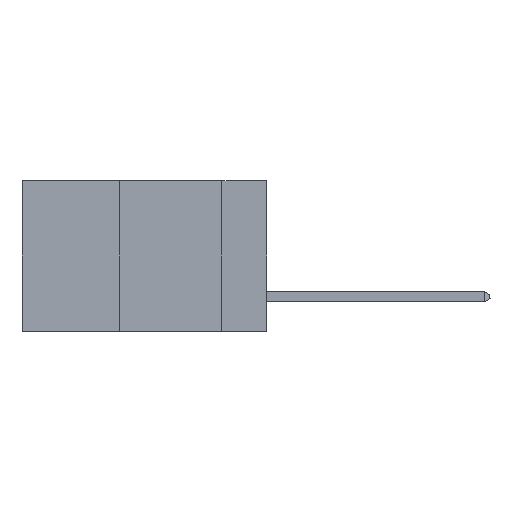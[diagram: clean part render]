
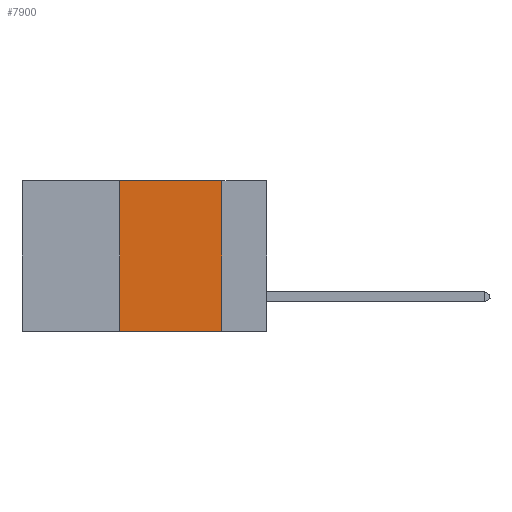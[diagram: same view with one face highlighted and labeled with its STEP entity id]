
A CAD part, left-side view. The second image highlights one B-rep face of the part: STEP entity #7900.
In plain terms, the highlighted planar face has unit normal (-1, 0, 0).
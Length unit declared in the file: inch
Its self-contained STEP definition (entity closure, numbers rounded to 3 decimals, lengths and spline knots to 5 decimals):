
#352 = DIRECTION ( 'NONE',  ( 0., -1., 0. ) ) ;
#360 = ORIENTED_EDGE ( 'NONE', *, *, #14036, .F. ) ;
#533 = LINE ( 'NONE', #4120, #10003 ) ;
#816 = VECTOR ( 'NONE', #3423, 39.37008 ) ;
#871 = EDGE_CURVE ( 'NONE', #8733, #17433, #17259, .T. ) ;
#1996 = CARTESIAN_POINT ( 'NONE',  ( 0., 0.11, 0. ) ) ;
#3182 = LINE ( 'NONE', #10126, #15303 ) ;
#3423 = DIRECTION ( 'NONE',  ( 0., 0., -1. ) ) ;
#3440 = CARTESIAN_POINT ( 'NONE',  ( 0., 0.36, -0.37 ) ) ;
#3669 = DIRECTION ( 'NONE',  ( 1., 0., 0. ) ) ;
#3854 = DIRECTION ( 'NONE',  ( 0., 0., -1. ) ) ;
#4120 = CARTESIAN_POINT ( 'NONE',  ( 0., 0.6, 0. ) ) ;
#4350 = DIRECTION ( 'NONE',  ( 0., -1., 0. ) ) ;
#4453 = CARTESIAN_POINT ( 'NONE',  ( 0., 0.11, 0. ) ) ;
#5924 = EDGE_LOOP ( 'NONE', ( #10846, #360, #6658, #10600 ) ) ;
#6421 = CARTESIAN_POINT ( 'NONE',  ( 0., 0.36, 0. ) ) ;
#6550 = EDGE_CURVE ( 'NONE', #15866, #17433, #3182, .T. ) ;
#6658 = ORIENTED_EDGE ( 'NONE', *, *, #17776, .F. ) ;
#7900 = ADVANCED_FACE ( 'NONE', ( #15439 ), #10641, .F. ) ;
#8733 = VERTEX_POINT ( 'NONE', #4453 ) ;
#9404 = VERTEX_POINT ( 'NONE', #10119 ) ;
#9426 = VECTOR ( 'NONE', #12469, 39.37008 ) ;
#9882 = LINE ( 'NONE', #6421, #9426 ) ;
#10003 = VECTOR ( 'NONE', #4350, 39.37008 ) ;
#10119 = CARTESIAN_POINT ( 'NONE',  ( 0., 0.36, 0. ) ) ;
#10126 = CARTESIAN_POINT ( 'NONE',  ( 0., 0.6, -0.37 ) ) ;
#10600 = ORIENTED_EDGE ( 'NONE', *, *, #6550, .T. ) ;
#10641 = PLANE ( 'NONE',  #13377 ) ;
#10846 = ORIENTED_EDGE ( 'NONE', *, *, #871, .F. ) ;
#12046 = CARTESIAN_POINT ( 'NONE',  ( 0., 0.6, 0. ) ) ;
#12469 = DIRECTION ( 'NONE',  ( 0., 0., 1. ) ) ;
#13377 = AXIS2_PLACEMENT_3D ( 'NONE', #12046, #3669, #3854 ) ;
#14036 = EDGE_CURVE ( 'NONE', #9404, #8733, #533, .T. ) ;
#15303 = VECTOR ( 'NONE', #352, 39.37008 ) ;
#15439 = FACE_OUTER_BOUND ( 'NONE', #5924, .T. ) ;
#15866 = VERTEX_POINT ( 'NONE', #3440 ) ;
#15991 = CARTESIAN_POINT ( 'NONE',  ( 0., 0.11, -0.37 ) ) ;
#17259 = LINE ( 'NONE', #1996, #816 ) ;
#17433 = VERTEX_POINT ( 'NONE', #15991 ) ;
#17776 = EDGE_CURVE ( 'NONE', #15866, #9404, #9882, .T. ) ;
